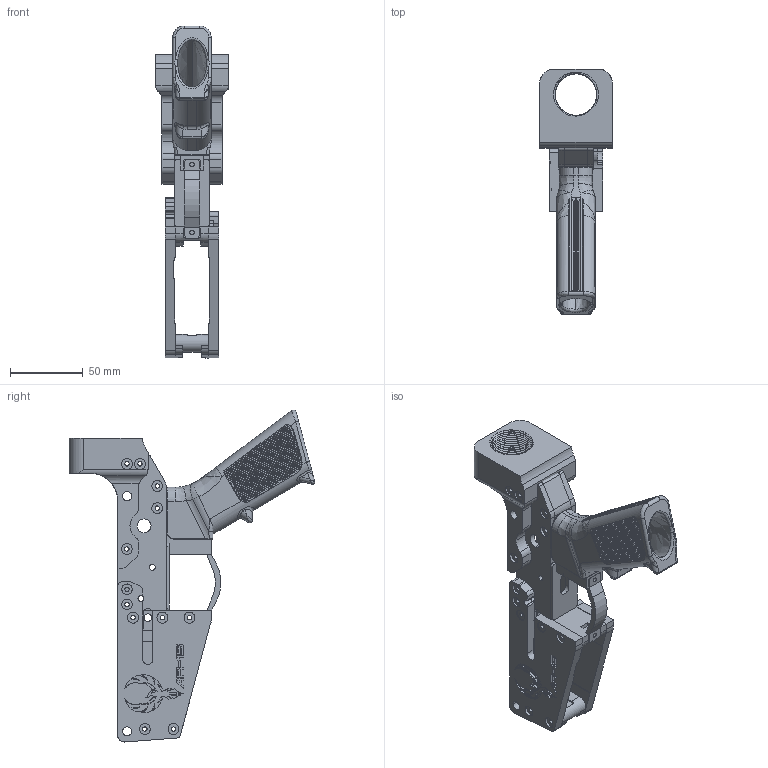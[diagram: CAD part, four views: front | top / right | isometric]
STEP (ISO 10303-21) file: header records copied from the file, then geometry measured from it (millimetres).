
FILE_DESCRIPTION (( 'STEP AP214' ), '1' );
FILE_NAME ('Firebolt_5.56_Standard.STEP', '2020-12-05T18:53:13', ( '' ), ( '' ), 'SwSTEP 2.0', 'SolidWorks 2020', '' );
FILE_SCHEMA (( 'AUTOMOTIVE_DESIGN' ));
Length unit declared in the file: millimetre
Products named in the file (12): Firebolt_Mag_Well_Front; Firebolt_Pistol_Grip; Firebolt_Mag_Well_Rear; Firebolt_Grip_Part; Firebolt_Mag_Well_Left; Firebolt_Trigger_Guard; Firebolt_Side_Left; Firebolt_Side_Right; Firebolt_5.56_Standard; Firebolt_Mag_Well_Right; Firebolt_Fire_Control_Well_Bottom; Firebolt_Buffer_Tower
Assembly tree (11 placements, depth 2):
  Firebolt_5.56_Standard
    Firebolt_Buffer_Tower
    Firebolt_Side_Left
    Firebolt_Side_Right
    Firebolt_Grip_Part
    Firebolt_Pistol_Grip
    Firebolt_Fire_Control_Well_Bottom
    Firebolt_Trigger_Guard
    Firebolt_Mag_Well_Rear
    Firebolt_Mag_Well_Right
    Firebolt_Mag_Well_Left
    Firebolt_Mag_Well_Front
Bounding box: 50 x 169.01 x 228.65 mm (x, y, z)
Volume: 253500.5 mm3; surface area: 116360.2 mm2
Topology: 11 solids, 11 shells, 7823 faces, 17166 edges, 10902 vertices
Faces by surface type: plane 7195, cylinder 456, bspline 168, cone 4
Entity records: 249844 total; most frequent: CARTESIAN_POINT 84440, ORIENTED_EDGE 34318, DIRECTION 29666, EDGE_CURVE 17159, VECTOR 12826, LINE 12826, VERTEX_POINT 10902, EDGE_LOOP 9517
